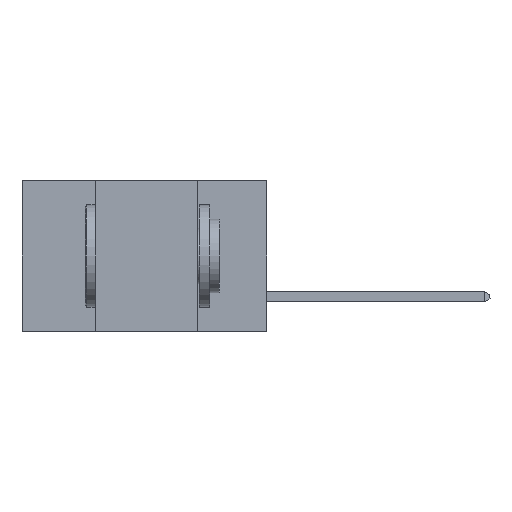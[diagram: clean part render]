
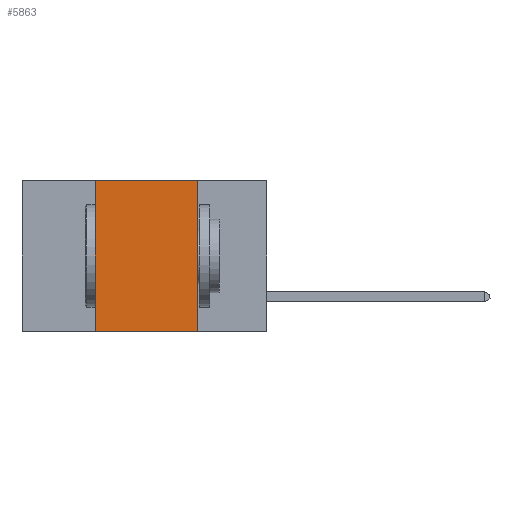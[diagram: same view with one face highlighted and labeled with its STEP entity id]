
A CAD part, left-side view. The second image highlights one B-rep face of the part: STEP entity #5863.
In plain terms, the highlighted planar face has unit normal (-1, 0, 0).
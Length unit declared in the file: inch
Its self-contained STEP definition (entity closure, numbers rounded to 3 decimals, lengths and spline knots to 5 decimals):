
#281 = VERTEX_POINT ( 'NONE', #1586 ) ;
#535 = ORIENTED_EDGE ( 'NONE', *, *, #1614, .F. ) ;
#712 = CARTESIAN_POINT ( 'NONE',  ( 0., 0.6, -0.37 ) ) ;
#743 = VERTEX_POINT ( 'NONE', #3855 ) ;
#770 = FACE_OUTER_BOUND ( 'NONE', #5036, .T. ) ;
#776 = CARTESIAN_POINT ( 'NONE',  ( 0., 0.6, 0. ) ) ;
#1586 = CARTESIAN_POINT ( 'NONE',  ( 0., 0.42, -0.37 ) ) ;
#1614 = EDGE_CURVE ( 'NONE', #281, #2868, #9189, .T. ) ;
#2254 = PLANE ( 'NONE',  #8418 ) ;
#2868 = VERTEX_POINT ( 'NONE', #5179 ) ;
#3033 = LINE ( 'NONE', #7059, #3714 ) ;
#3589 = LINE ( 'NONE', #712, #5682 ) ;
#3709 = CARTESIAN_POINT ( 'NONE',  ( 0., 0.17, 0. ) ) ;
#3714 = VECTOR ( 'NONE', #4101, 39.37008 ) ;
#3855 = CARTESIAN_POINT ( 'NONE',  ( 0., 0.17, -0.37 ) ) ;
#4101 = DIRECTION ( 'NONE',  ( 0., -1., 0. ) ) ;
#4309 = ORIENTED_EDGE ( 'NONE', *, *, #5039, .F. ) ;
#5036 = EDGE_LOOP ( 'NONE', ( #4309, #7739, #535, #7381 ) ) ;
#5039 = EDGE_CURVE ( 'NONE', #5946, #743, #8778, .T. ) ;
#5158 = CARTESIAN_POINT ( 'NONE',  ( 0., 0.42, 0. ) ) ;
#5179 = CARTESIAN_POINT ( 'NONE',  ( 0., 0.42, 0. ) ) ;
#5682 = VECTOR ( 'NONE', #5869, 39.37008 ) ;
#5863 = ADVANCED_FACE ( 'NONE', ( #770 ), #2254, .F. ) ;
#5869 = DIRECTION ( 'NONE',  ( 0., -1., 0. ) ) ;
#5925 = DIRECTION ( 'NONE',  ( 0., 0., 1. ) ) ;
#5946 = VERTEX_POINT ( 'NONE', #3709 ) ;
#6714 = DIRECTION ( 'NONE',  ( 1., 0., 0. ) ) ;
#7001 = DIRECTION ( 'NONE',  ( 0., 0., -1. ) ) ;
#7059 = CARTESIAN_POINT ( 'NONE',  ( 0., 0.6, 0. ) ) ;
#7356 = VECTOR ( 'NONE', #7001, 39.37008 ) ;
#7381 = ORIENTED_EDGE ( 'NONE', *, *, #9392, .T. ) ;
#7739 = ORIENTED_EDGE ( 'NONE', *, *, #8574, .F. ) ;
#8109 = DIRECTION ( 'NONE',  ( 0., 0., -1. ) ) ;
#8361 = CARTESIAN_POINT ( 'NONE',  ( 0., 0.17, 0. ) ) ;
#8418 = AXIS2_PLACEMENT_3D ( 'NONE', #776, #6714, #8109 ) ;
#8574 = EDGE_CURVE ( 'NONE', #2868, #5946, #3033, .T. ) ;
#8778 = LINE ( 'NONE', #8361, #7356 ) ;
#8957 = VECTOR ( 'NONE', #5925, 39.37008 ) ;
#9189 = LINE ( 'NONE', #5158, #8957 ) ;
#9392 = EDGE_CURVE ( 'NONE', #281, #743, #3589, .T. ) ;
